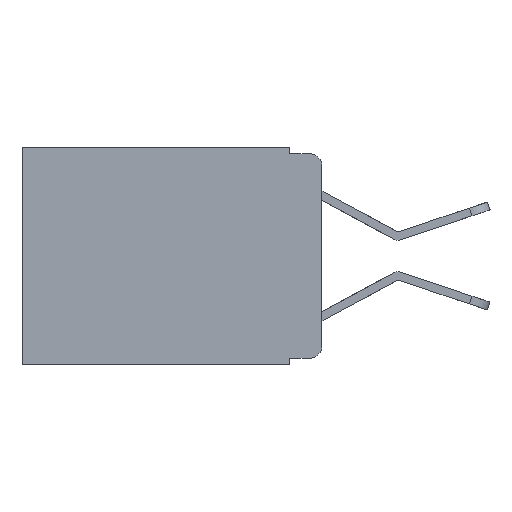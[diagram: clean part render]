
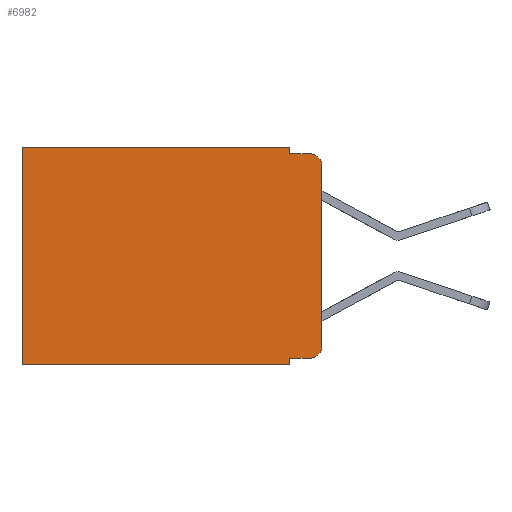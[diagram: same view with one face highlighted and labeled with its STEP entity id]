
A CAD part, left-side view. The second image highlights one B-rep face of the part: STEP entity #6982.
In plain terms, the highlighted planar face has unit normal (-1, 0, 0).
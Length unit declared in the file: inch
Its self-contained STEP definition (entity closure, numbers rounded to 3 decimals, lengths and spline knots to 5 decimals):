
#20 = LINE ( 'NONE', #1861, #6781 ) ;
#136 = DIRECTION ( 'NONE',  ( 0., -1., 0. ) ) ;
#275 = CARTESIAN_POINT ( 'NONE',  ( 0.298, 0.473, 0. ) ) ;
#746 = PLANE ( 'NONE',  #7544 ) ;
#1086 = CARTESIAN_POINT ( 'NONE',  ( 0.298, 0.051, -0.01 ) ) ;
#1216 = EDGE_CURVE ( 'NONE', #6333, #7994, #7071, .T. ) ;
#1396 = VERTEX_POINT ( 'NONE', #275 ) ;
#1499 = EDGE_CURVE ( 'NONE', #7994, #7917, #11061, .T. ) ;
#1650 = LINE ( 'NONE', #9431, #10642 ) ;
#1694 = LINE ( 'NONE', #4440, #7754 ) ;
#1751 = DIRECTION ( 'NONE',  ( 1., 0., 0. ) ) ;
#1816 = DIRECTION ( 'NONE',  ( -1., 0., 0. ) ) ;
#1817 = VECTOR ( 'NONE', #6524, 39.37008 ) ;
#1861 = CARTESIAN_POINT ( 'NONE',  ( 0.298, 0., 0. ) ) ;
#1892 = AXIS2_PLACEMENT_3D ( 'NONE', #9566, #4306, #10352 ) ;
#1949 = ORIENTED_EDGE ( 'NONE', *, *, #3420, .F. ) ;
#1981 = VERTEX_POINT ( 'NONE', #6230 ) ;
#2236 = LINE ( 'NONE', #5718, #2509 ) ;
#2240 = CARTESIAN_POINT ( 'NONE',  ( 0.298, 0.051, -0.333 ) ) ;
#2251 = CARTESIAN_POINT ( 'NONE',  ( 0.298, 0.051, -0.01 ) ) ;
#2383 = LINE ( 'NONE', #8248, #6583 ) ;
#2509 = VECTOR ( 'NONE', #4803, 39.37008 ) ;
#2759 = DIRECTION ( 'NONE',  ( 0., 0., -1. ) ) ;
#3278 = EDGE_LOOP ( 'NONE', ( #9662, #5031, #10154, #6032, #11040, #3515, #1949, #6579, #7439, #9029 ) ) ;
#3420 = EDGE_CURVE ( 'NONE', #5598, #1981, #1694, .T. ) ;
#3515 = ORIENTED_EDGE ( 'NONE', *, *, #7195, .T. ) ;
#3936 = AXIS2_PLACEMENT_3D ( 'NONE', #7263, #1816, #8051 ) ;
#4182 = DIRECTION ( 'NONE',  ( 0., 0., -1. ) ) ;
#4306 = DIRECTION ( 'NONE',  ( -1., 0., 0. ) ) ;
#4440 = CARTESIAN_POINT ( 'NONE',  ( 0.298, 0., -0.343 ) ) ;
#4444 = CARTESIAN_POINT ( 'NONE',  ( 0.298, 0.051, 0. ) ) ;
#4745 = VERTEX_POINT ( 'NONE', #4444 ) ;
#4803 = DIRECTION ( 'NONE',  ( 0., 0., -1. ) ) ;
#4948 = DIRECTION ( 'NONE',  ( 0., 1., 0. ) ) ;
#5025 = EDGE_CURVE ( 'NONE', #4745, #1396, #5037, .T. ) ;
#5031 = ORIENTED_EDGE ( 'NONE', *, *, #7904, .T. ) ;
#5037 = LINE ( 'NONE', #5104, #7716 ) ;
#5040 = FACE_OUTER_BOUND ( 'NONE', #3278, .T. ) ;
#5104 = CARTESIAN_POINT ( 'NONE',  ( 0.298, 0., 0. ) ) ;
#5224 = CARTESIAN_POINT ( 'NONE',  ( 0.298, 0., -0.313 ) ) ;
#5326 = CIRCLE ( 'NONE', #1892, 0.02 ) ;
#5427 = CARTESIAN_POINT ( 'NONE',  ( 0.298, 0.051, -0.343 ) ) ;
#5598 = VERTEX_POINT ( 'NONE', #5427 ) ;
#5718 = CARTESIAN_POINT ( 'NONE',  ( 0.298, 0.473, 0. ) ) ;
#6032 = ORIENTED_EDGE ( 'NONE', *, *, #7836, .F. ) ;
#6184 = CARTESIAN_POINT ( 'NONE',  ( 0.298, 0., 0. ) ) ;
#6230 = CARTESIAN_POINT ( 'NONE',  ( 0.298, 0.473, -0.343 ) ) ;
#6333 = VERTEX_POINT ( 'NONE', #11098 ) ;
#6516 = VECTOR ( 'NONE', #136, 39.37008 ) ;
#6524 = DIRECTION ( 'NONE',  ( 0., -1., 0. ) ) ;
#6579 = ORIENTED_EDGE ( 'NONE', *, *, #7678, .F. ) ;
#6583 = VECTOR ( 'NONE', #8287, 39.37008 ) ;
#6781 = VECTOR ( 'NONE', #2759, 39.37008 ) ;
#6982 = ADVANCED_FACE ( 'NONE', ( #5040 ), #746, .F. ) ;
#7071 = LINE ( 'NONE', #2240, #6516 ) ;
#7195 = EDGE_CURVE ( 'NONE', #1396, #1981, #2236, .T. ) ;
#7225 = VERTEX_POINT ( 'NONE', #10063 ) ;
#7263 = CARTESIAN_POINT ( 'NONE',  ( 0.298, 0.02, -0.313 ) ) ;
#7439 = ORIENTED_EDGE ( 'NONE', *, *, #1216, .T. ) ;
#7544 = AXIS2_PLACEMENT_3D ( 'NONE', #6184, #1751, #8044 ) ;
#7678 = EDGE_CURVE ( 'NONE', #6333, #5598, #2383, .T. ) ;
#7697 = EDGE_CURVE ( 'NONE', #8236, #7225, #10769, .T. ) ;
#7716 = VECTOR ( 'NONE', #10768, 39.37008 ) ;
#7754 = VECTOR ( 'NONE', #4948, 39.37008 ) ;
#7836 = EDGE_CURVE ( 'NONE', #4745, #8236, #1650, .T. ) ;
#7904 = EDGE_CURVE ( 'NONE', #8111, #7225, #5326, .T. ) ;
#7917 = VERTEX_POINT ( 'NONE', #5224 ) ;
#7994 = VERTEX_POINT ( 'NONE', #8016 ) ;
#8016 = CARTESIAN_POINT ( 'NONE',  ( 0.298, 0.02, -0.333 ) ) ;
#8044 = DIRECTION ( 'NONE',  ( 0., 0., -1. ) ) ;
#8051 = DIRECTION ( 'NONE',  ( 0., 0., -1. ) ) ;
#8111 = VERTEX_POINT ( 'NONE', #9768 ) ;
#8236 = VERTEX_POINT ( 'NONE', #2251 ) ;
#8248 = CARTESIAN_POINT ( 'NONE',  ( 0.298, 0.051, 0. ) ) ;
#8287 = DIRECTION ( 'NONE',  ( 0., 0., -1. ) ) ;
#9029 = ORIENTED_EDGE ( 'NONE', *, *, #1499, .T. ) ;
#9431 = CARTESIAN_POINT ( 'NONE',  ( 0.298, 0.051, 0. ) ) ;
#9566 = CARTESIAN_POINT ( 'NONE',  ( 0.298, 0.02, -0.03 ) ) ;
#9662 = ORIENTED_EDGE ( 'NONE', *, *, #11336, .F. ) ;
#9768 = CARTESIAN_POINT ( 'NONE',  ( 0.298, 0., -0.03 ) ) ;
#10063 = CARTESIAN_POINT ( 'NONE',  ( 0.298, 0.02, -0.01 ) ) ;
#10154 = ORIENTED_EDGE ( 'NONE', *, *, #7697, .F. ) ;
#10352 = DIRECTION ( 'NONE',  ( 0., 0., -1. ) ) ;
#10642 = VECTOR ( 'NONE', #4182, 39.37008 ) ;
#10768 = DIRECTION ( 'NONE',  ( 0., 1., 0. ) ) ;
#10769 = LINE ( 'NONE', #1086, #1817 ) ;
#11040 = ORIENTED_EDGE ( 'NONE', *, *, #5025, .T. ) ;
#11061 = CIRCLE ( 'NONE', #3936, 0.02 ) ;
#11098 = CARTESIAN_POINT ( 'NONE',  ( 0.298, 0.051, -0.333 ) ) ;
#11336 = EDGE_CURVE ( 'NONE', #8111, #7917, #20, .T. ) ;
